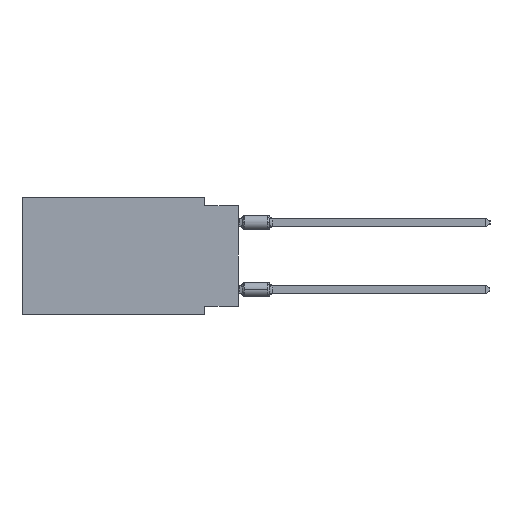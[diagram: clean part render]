
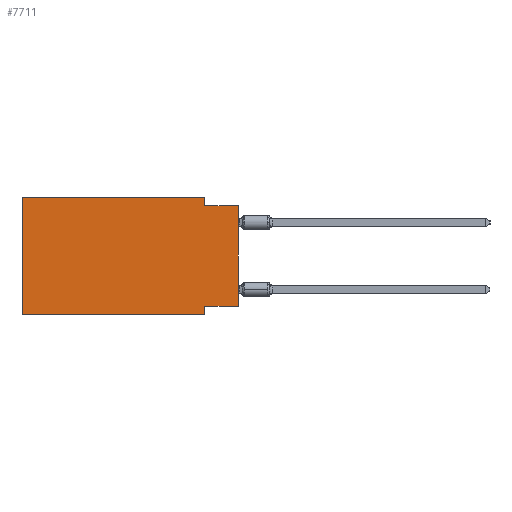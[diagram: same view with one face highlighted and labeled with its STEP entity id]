
A CAD part, left-side view. The second image highlights one B-rep face of the part: STEP entity #7711.
In plain terms, the highlighted planar face has unit normal (-1, 0, 0).
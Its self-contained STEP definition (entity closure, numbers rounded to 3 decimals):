
#1066 = EDGE_CURVE ( 'NONE', #40085, #30941, #43196, .T. ) ;
#1304 = EDGE_CURVE ( 'NONE', #17097, #40085, #21120, .T. ) ;
#2587 = CARTESIAN_POINT ( 'NONE',  ( 0., 16.383, -8.89 ) ) ;
#3511 = VERTEX_POINT ( 'NONE', #13337 ) ;
#3523 = VERTEX_POINT ( 'NONE', #13111 ) ;
#3755 = DIRECTION ( 'NONE',  ( 0., -1., 0. ) ) ;
#5173 = CARTESIAN_POINT ( 'NONE',  ( 0., 2.54, -8.89 ) ) ;
#5458 = VECTOR ( 'NONE', #13827, 1000. ) ;
#7249 = CARTESIAN_POINT ( 'NONE',  ( 0., 16.383, 0. ) ) ;
#7711 = ADVANCED_FACE ( 'NONE', ( #13524 ), #39796, .F. ) ;
#10019 = DIRECTION ( 'NONE',  ( 0., 0., 1. ) ) ;
#12173 = ORIENTED_EDGE ( 'NONE', *, *, #22588, .F. ) ;
#12855 = DIRECTION ( 'NONE',  ( 0., 1., 0. ) ) ;
#13104 = CARTESIAN_POINT ( 'NONE',  ( 0., 0., 0. ) ) ;
#13111 = CARTESIAN_POINT ( 'NONE',  ( 0., 2.54, -8.255 ) ) ;
#13337 = CARTESIAN_POINT ( 'NONE',  ( 0., 16.383, -8.89 ) ) ;
#13524 = FACE_OUTER_BOUND ( 'NONE', #14341, .T. ) ;
#13827 = DIRECTION ( 'NONE',  ( 0., -1., 0. ) ) ;
#13924 = CARTESIAN_POINT ( 'NONE',  ( 0., 16.383, 0. ) ) ;
#14327 = CARTESIAN_POINT ( 'NONE',  ( 0., 2.54, -8.89 ) ) ;
#14341 = EDGE_LOOP ( 'NONE', ( #29633, #24675, #26705, #12173, #28122, #20630, #38755, #25690 ) ) ;
#15960 = LINE ( 'NONE', #29406, #29179 ) ;
#17097 = VERTEX_POINT ( 'NONE', #21127 ) ;
#17232 = VECTOR ( 'NONE', #39669, 1000. ) ;
#19549 = VECTOR ( 'NONE', #34571, 1000. ) ;
#19896 = VERTEX_POINT ( 'NONE', #43097 ) ;
#19933 = DIRECTION ( 'NONE',  ( 0., 0., -1. ) ) ;
#20047 = VECTOR ( 'NONE', #36558, 1000. ) ;
#20630 = ORIENTED_EDGE ( 'NONE', *, *, #37609, .T. ) ;
#21120 = LINE ( 'NONE', #41627, #19549 ) ;
#21127 = CARTESIAN_POINT ( 'NONE',  ( 0., 2.54, 0. ) ) ;
#21328 = DIRECTION ( 'NONE',  ( 0., 0., -1. ) ) ;
#22588 = EDGE_CURVE ( 'NONE', #34728, #17097, #31114, .T. ) ;
#23358 = CARTESIAN_POINT ( 'NONE',  ( 0., 0., -0.635 ) ) ;
#24215 = EDGE_CURVE ( 'NONE', #3523, #28274, #41822, .T. ) ;
#24675 = ORIENTED_EDGE ( 'NONE', *, *, #1066, .F. ) ;
#25690 = ORIENTED_EDGE ( 'NONE', *, *, #27277, .F. ) ;
#26705 = ORIENTED_EDGE ( 'NONE', *, *, #1304, .F. ) ;
#27277 = EDGE_CURVE ( 'NONE', #19896, #3523, #15960, .T. ) ;
#27945 = VECTOR ( 'NONE', #21328, 1000. ) ;
#28122 = ORIENTED_EDGE ( 'NONE', *, *, #29047, .F. ) ;
#28274 = VERTEX_POINT ( 'NONE', #14327 ) ;
#29047 = EDGE_CURVE ( 'NONE', #3511, #34728, #33450, .T. ) ;
#29179 = VECTOR ( 'NONE', #12855, 1000. ) ;
#29406 = CARTESIAN_POINT ( 'NONE',  ( 0., 0., -8.255 ) ) ;
#29633 = ORIENTED_EDGE ( 'NONE', *, *, #41760, .T. ) ;
#30020 = VECTOR ( 'NONE', #3755, 1000. ) ;
#30941 = VERTEX_POINT ( 'NONE', #42626 ) ;
#31114 = LINE ( 'NONE', #13924, #30020 ) ;
#32419 = AXIS2_PLACEMENT_3D ( 'NONE', #37131, #37343, #19933 ) ;
#32793 = CARTESIAN_POINT ( 'NONE',  ( 0., 2.54, -0.635 ) ) ;
#32820 = LINE ( 'NONE', #2587, #17232 ) ;
#33450 = LINE ( 'NONE', #33896, #20047 ) ;
#33896 = CARTESIAN_POINT ( 'NONE',  ( 0., 16.383, 0. ) ) ;
#34571 = DIRECTION ( 'NONE',  ( 0., 0., -1. ) ) ;
#34728 = VERTEX_POINT ( 'NONE', #7249 ) ;
#36558 = DIRECTION ( 'NONE',  ( 0., 0., 1. ) ) ;
#37131 = CARTESIAN_POINT ( 'NONE',  ( 0., 16.383, 0. ) ) ;
#37343 = DIRECTION ( 'NONE',  ( 1., 0., 0. ) ) ;
#37609 = EDGE_CURVE ( 'NONE', #3511, #28274, #32820, .T. ) ;
#38755 = ORIENTED_EDGE ( 'NONE', *, *, #24215, .F. ) ;
#39050 = VECTOR ( 'NONE', #10019, 1000. ) ;
#39669 = DIRECTION ( 'NONE',  ( 0., -1., 0. ) ) ;
#39796 = PLANE ( 'NONE',  #32419 ) ;
#40037 = LINE ( 'NONE', #13104, #39050 ) ;
#40085 = VERTEX_POINT ( 'NONE', #32793 ) ;
#41627 = CARTESIAN_POINT ( 'NONE',  ( 0., 2.54, 0. ) ) ;
#41760 = EDGE_CURVE ( 'NONE', #19896, #30941, #40037, .T. ) ;
#41822 = LINE ( 'NONE', #5173, #27945 ) ;
#42626 = CARTESIAN_POINT ( 'NONE',  ( 0., 0., -0.635 ) ) ;
#43097 = CARTESIAN_POINT ( 'NONE',  ( 0., 0., -8.255 ) ) ;
#43196 = LINE ( 'NONE', #23358, #5458 ) ;
